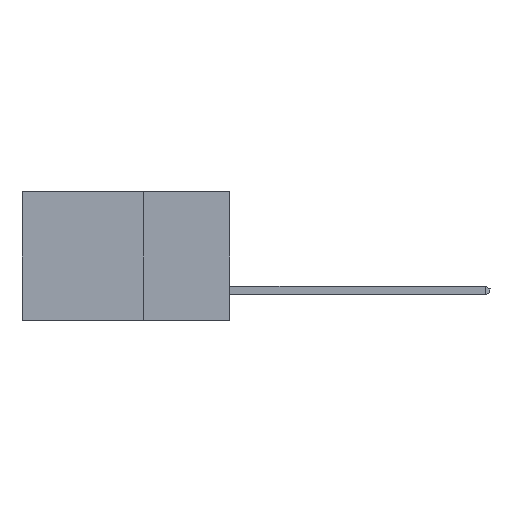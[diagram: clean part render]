
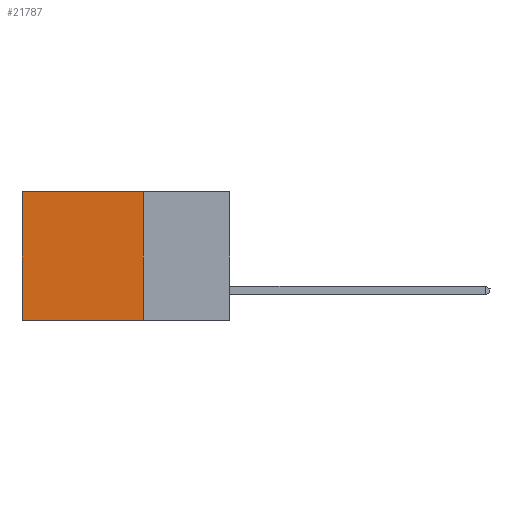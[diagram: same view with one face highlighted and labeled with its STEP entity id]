
A CAD part, left-side view. The second image highlights one B-rep face of the part: STEP entity #21787.
In plain terms, the highlighted planar face has unit normal (-1, 0, 0).
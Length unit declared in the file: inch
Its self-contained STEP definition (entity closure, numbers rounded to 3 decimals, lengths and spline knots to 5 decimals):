
#366 = CARTESIAN_POINT ( 'NONE',  ( 0.2615, 0.6, -0.37 ) ) ;
#515 = VERTEX_POINT ( 'NONE', #3626 ) ;
#3626 = CARTESIAN_POINT ( 'NONE',  ( 0.2615, 0.25, -0.37 ) ) ;
#3897 = VERTEX_POINT ( 'NONE', #11343 ) ;
#4321 = EDGE_CURVE ( 'NONE', #3897, #15896, #4570, .T. ) ;
#4570 = LINE ( 'NONE', #18068, #5845 ) ;
#5032 = AXIS2_PLACEMENT_3D ( 'NONE', #19320, #12671, #17129 ) ;
#5845 = VECTOR ( 'NONE', #16420, 39.37008 ) ;
#6033 = PLANE ( 'NONE',  #5032 ) ;
#6056 = CARTESIAN_POINT ( 'NONE',  ( 0.2615, 0.25, -0.37 ) ) ;
#8139 = VECTOR ( 'NONE', #18101, 39.37008 ) ;
#8811 = CARTESIAN_POINT ( 'NONE',  ( 0.2615, 0.25, 0. ) ) ;
#9135 = VECTOR ( 'NONE', #21864, 39.37008 ) ;
#9869 = EDGE_CURVE ( 'NONE', #515, #15896, #18431, .T. ) ;
#11079 = EDGE_LOOP ( 'NONE', ( #14848, #14842, #20958, #16453 ) ) ;
#11343 = CARTESIAN_POINT ( 'NONE',  ( 0.2615, 0.6, 0. ) ) ;
#11581 = LINE ( 'NONE', #18120, #13109 ) ;
#12671 = DIRECTION ( 'NONE',  ( 1., 0., 0. ) ) ;
#13109 = VECTOR ( 'NONE', #18338, 39.37008 ) ;
#14842 = ORIENTED_EDGE ( 'NONE', *, *, #9869, .F. ) ;
#14848 = ORIENTED_EDGE ( 'NONE', *, *, #4321, .T. ) ;
#14892 = CARTESIAN_POINT ( 'NONE',  ( 0.2615, 0.25, -0.37 ) ) ;
#15477 = FACE_OUTER_BOUND ( 'NONE', #11079, .T. ) ;
#15896 = VERTEX_POINT ( 'NONE', #366 ) ;
#16180 = EDGE_CURVE ( 'NONE', #19389, #3897, #11581, .T. ) ;
#16420 = DIRECTION ( 'NONE',  ( 0., 0., -1. ) ) ;
#16453 = ORIENTED_EDGE ( 'NONE', *, *, #16180, .T. ) ;
#17129 = DIRECTION ( 'NONE',  ( 0., 0., -1. ) ) ;
#18068 = CARTESIAN_POINT ( 'NONE',  ( 0.2615, 0.6, -0.37 ) ) ;
#18101 = DIRECTION ( 'NONE',  ( 0., 0., -1. ) ) ;
#18120 = CARTESIAN_POINT ( 'NONE',  ( 0.2615, 0.25, 0. ) ) ;
#18338 = DIRECTION ( 'NONE',  ( 0., 1., 0. ) ) ;
#18431 = LINE ( 'NONE', #14892, #9135 ) ;
#19320 = CARTESIAN_POINT ( 'NONE',  ( 0.2615, 0.25, -0.37 ) ) ;
#19389 = VERTEX_POINT ( 'NONE', #8811 ) ;
#19504 = EDGE_CURVE ( 'NONE', #19389, #515, #19666, .T. ) ;
#19666 = LINE ( 'NONE', #6056, #8139 ) ;
#20958 = ORIENTED_EDGE ( 'NONE', *, *, #19504, .F. ) ;
#21787 = ADVANCED_FACE ( 'NONE', ( #15477 ), #6033, .F. ) ;
#21864 = DIRECTION ( 'NONE',  ( 0., 1., 0. ) ) ;
